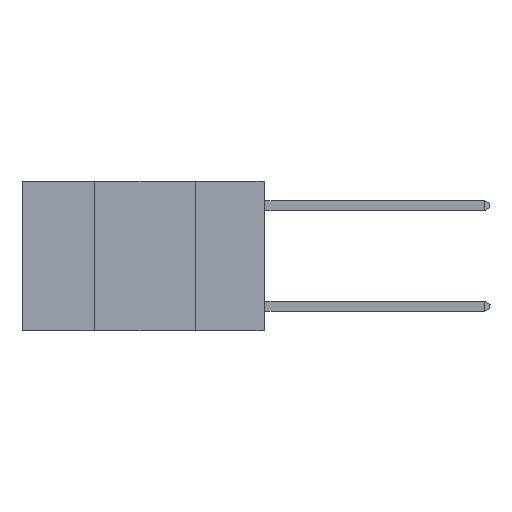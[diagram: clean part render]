
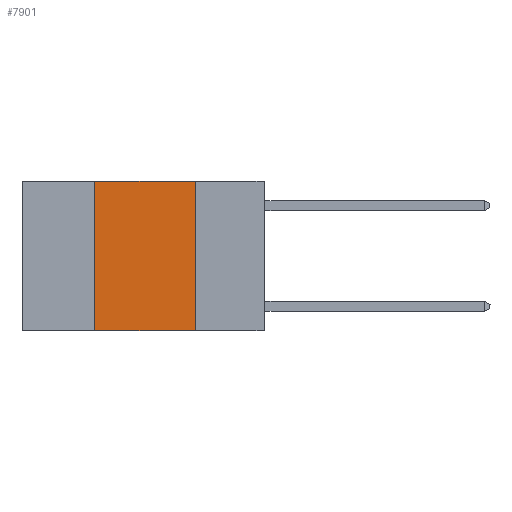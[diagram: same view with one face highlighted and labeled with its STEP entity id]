
A CAD part, left-side view. The second image highlights one B-rep face of the part: STEP entity #7901.
In plain terms, the highlighted planar face has unit normal (-1, 0, 0).
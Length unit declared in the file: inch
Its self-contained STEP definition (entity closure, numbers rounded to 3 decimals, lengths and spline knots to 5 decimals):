
#41 = ORIENTED_EDGE ( 'NONE', *, *, #5386, .F. ) ;
#59 = CARTESIAN_POINT ( 'NONE',  ( 0., 0.42, 0. ) ) ;
#207 = VERTEX_POINT ( 'NONE', #10271 ) ;
#310 = CARTESIAN_POINT ( 'NONE',  ( 0., 0.17, 0. ) ) ;
#407 = VECTOR ( 'NONE', #12761, 39.37008 ) ;
#431 = CARTESIAN_POINT ( 'NONE',  ( 0., 0.42, -0.37 ) ) ;
#663 = DIRECTION ( 'NONE',  ( 1., 0., 0. ) ) ;
#1361 = DIRECTION ( 'NONE',  ( 0., 0., -1. ) ) ;
#1899 = CARTESIAN_POINT ( 'NONE',  ( 0., 0.42, 0. ) ) ;
#2763 = FACE_OUTER_BOUND ( 'NONE', #6965, .T. ) ;
#2819 = VERTEX_POINT ( 'NONE', #9376 ) ;
#3668 = VECTOR ( 'NONE', #8184, 39.37008 ) ;
#4101 = CARTESIAN_POINT ( 'NONE',  ( 0., 0.6, -0.37 ) ) ;
#5386 = EDGE_CURVE ( 'NONE', #2819, #207, #6628, .T. ) ;
#5531 = ORIENTED_EDGE ( 'NONE', *, *, #10173, .F. ) ;
#5837 = VERTEX_POINT ( 'NONE', #1899 ) ;
#6024 = LINE ( 'NONE', #59, #8796 ) ;
#6298 = VECTOR ( 'NONE', #1361, 39.37008 ) ;
#6628 = LINE ( 'NONE', #310, #6298 ) ;
#6965 = EDGE_LOOP ( 'NONE', ( #41, #5531, #8251, #10883 ) ) ;
#7252 = DIRECTION ( 'NONE',  ( 0., 0., 1. ) ) ;
#7862 = DIRECTION ( 'NONE',  ( 0., 0., -1. ) ) ;
#7901 = ADVANCED_FACE ( 'NONE', ( #2763 ), #12752, .F. ) ;
#8039 = AXIS2_PLACEMENT_3D ( 'NONE', #9834, #663, #7862 ) ;
#8184 = DIRECTION ( 'NONE',  ( 0., -1., 0. ) ) ;
#8251 = ORIENTED_EDGE ( 'NONE', *, *, #12973, .F. ) ;
#8625 = LINE ( 'NONE', #11809, #407 ) ;
#8796 = VECTOR ( 'NONE', #7252, 39.37008 ) ;
#9376 = CARTESIAN_POINT ( 'NONE',  ( 0., 0.17, 0. ) ) ;
#9403 = LINE ( 'NONE', #4101, #3668 ) ;
#9834 = CARTESIAN_POINT ( 'NONE',  ( 0., 0.6, 0. ) ) ;
#10173 = EDGE_CURVE ( 'NONE', #5837, #2819, #8625, .T. ) ;
#10271 = CARTESIAN_POINT ( 'NONE',  ( 0., 0.17, -0.37 ) ) ;
#10372 = EDGE_CURVE ( 'NONE', #12507, #207, #9403, .T. ) ;
#10883 = ORIENTED_EDGE ( 'NONE', *, *, #10372, .T. ) ;
#11809 = CARTESIAN_POINT ( 'NONE',  ( 0., 0.6, 0. ) ) ;
#12507 = VERTEX_POINT ( 'NONE', #431 ) ;
#12752 = PLANE ( 'NONE',  #8039 ) ;
#12761 = DIRECTION ( 'NONE',  ( 0., -1., 0. ) ) ;
#12973 = EDGE_CURVE ( 'NONE', #12507, #5837, #6024, .T. ) ;
